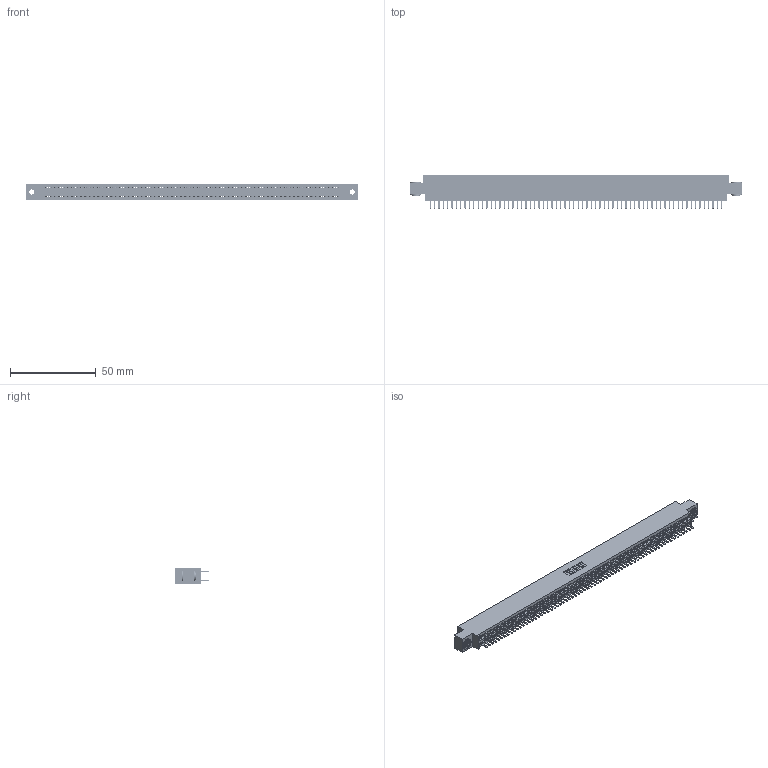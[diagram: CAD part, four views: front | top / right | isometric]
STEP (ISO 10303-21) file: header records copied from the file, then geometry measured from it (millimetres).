
FILE_DESCRIPTION (( 'STEP AP203' ), '1' );
FILE_NAME ('345-136-520-803.STEP', '2019-11-08T06:27:36', ( '' ), ( '' ), 'SwSTEP 2.0', 'SolidWorks 2016', '' );
FILE_SCHEMA (( 'CONFIG_CONTROL_DESIGN' ));
Length unit declared in the file: inch
Products named in the file (4): 345-250-002_345-250-002-102; 345-136-520-803; 345-292-001_345-293-120; 345 Part_0.170 Offset - 0.156 Dia-TH
Assembly tree (139 placements, depth 2):
  345-136-520-803
    345 Part_0.170 Offset - 0.156 Dia-TH
    345-292-001_345-293-120  x136
    345-250-002_345-250-002-102  x2
Bounding box: 193.93 x 19.68 x 9.4 mm (x, y, z)
Volume: 18926 mm3; surface area: 28700.6 mm2
Topology: 139 solids, 139 shells, 7512 faces, 21781 edges, 14154 vertices
Faces by surface type: plane 4854, cylinder 2650, cone 8
Entity records: 50750 total; most frequent: CARTESIAN_POINT 8471, ORIENTED_EDGE 8386, DIRECTION 7455, EDGE_CURVE 4193, VECTOR 3761, LINE 3761, VERTEX_POINT 2790, AXIS2_PLACEMENT_3D 1847
